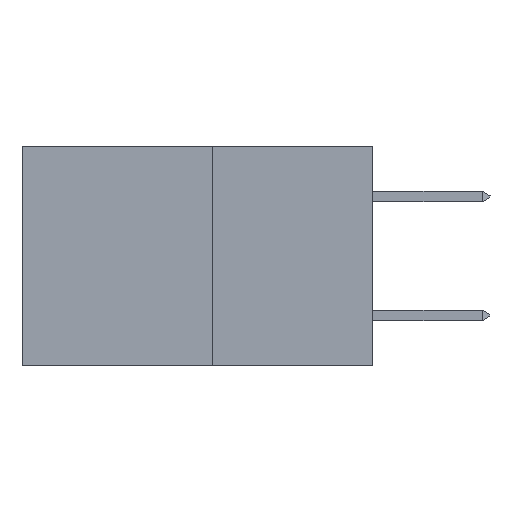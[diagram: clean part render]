
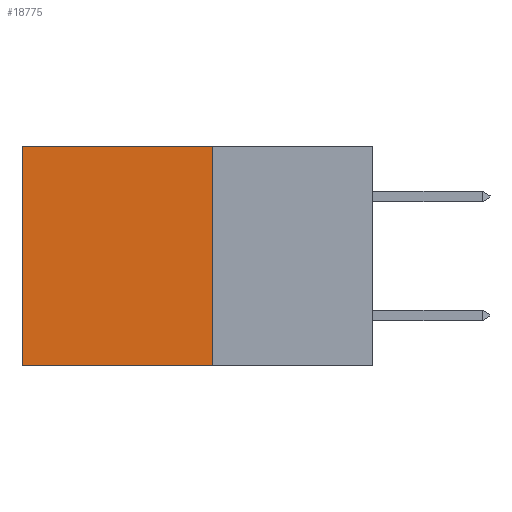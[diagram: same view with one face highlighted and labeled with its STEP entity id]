
A CAD part, left-side view. The second image highlights one B-rep face of the part: STEP entity #18775.
In plain terms, the highlighted planar face has unit normal (-1, 0, 0).
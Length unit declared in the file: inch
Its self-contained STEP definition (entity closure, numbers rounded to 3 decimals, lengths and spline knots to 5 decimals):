
#288 = AXIS2_PLACEMENT_3D ( 'NONE', #17967, #27277, #13423 ) ;
#622 = LINE ( 'NONE', #27732, #6665 ) ;
#1405 = EDGE_LOOP ( 'NONE', ( #4327, #21968, #26603, #13344 ) ) ;
#1466 = CARTESIAN_POINT ( 'NONE',  ( 0.277, 0.59, -0.37 ) ) ;
#2612 = VERTEX_POINT ( 'NONE', #11023 ) ;
#4327 = ORIENTED_EDGE ( 'NONE', *, *, #29177, .T. ) ;
#4987 = VECTOR ( 'NONE', #11175, 39.37008 ) ;
#5546 = VECTOR ( 'NONE', #26378, 39.37008 ) ;
#5677 = FACE_OUTER_BOUND ( 'NONE', #1405, .T. ) ;
#6189 = VERTEX_POINT ( 'NONE', #13771 ) ;
#6361 = VERTEX_POINT ( 'NONE', #23608 ) ;
#6665 = VECTOR ( 'NONE', #20857, 39.37008 ) ;
#9851 = DIRECTION ( 'NONE',  ( 0., 1., 0. ) ) ;
#11023 = CARTESIAN_POINT ( 'NONE',  ( 0.277, 0.27, -0.37 ) ) ;
#11074 = PLANE ( 'NONE',  #288 ) ;
#11175 = DIRECTION ( 'NONE',  ( 0., 0., -1. ) ) ;
#12424 = EDGE_CURVE ( 'NONE', #6189, #6361, #27071, .T. ) ;
#13344 = ORIENTED_EDGE ( 'NONE', *, *, #12424, .T. ) ;
#13423 = DIRECTION ( 'NONE',  ( 0., 0., -1. ) ) ;
#13771 = CARTESIAN_POINT ( 'NONE',  ( 0.277, 0.27, 0. ) ) ;
#15841 = CARTESIAN_POINT ( 'NONE',  ( 0.277, 0.27, -0.37 ) ) ;
#16478 = LINE ( 'NONE', #15841, #4987 ) ;
#17967 = CARTESIAN_POINT ( 'NONE',  ( 0.277, 0.27, -0.37 ) ) ;
#18775 = ADVANCED_FACE ( 'NONE', ( #5677 ), #11074, .F. ) ;
#18825 = EDGE_CURVE ( 'NONE', #6189, #2612, #16478, .T. ) ;
#20528 = EDGE_CURVE ( 'NONE', #2612, #22655, #24691, .T. ) ;
#20857 = DIRECTION ( 'NONE',  ( 0., 0., -1. ) ) ;
#20936 = VECTOR ( 'NONE', #9851, 39.37008 ) ;
#21968 = ORIENTED_EDGE ( 'NONE', *, *, #20528, .F. ) ;
#22655 = VERTEX_POINT ( 'NONE', #1466 ) ;
#23608 = CARTESIAN_POINT ( 'NONE',  ( 0.277, 0.59, 0. ) ) ;
#24691 = LINE ( 'NONE', #26483, #5546 ) ;
#26072 = CARTESIAN_POINT ( 'NONE',  ( 0.277, 0.27, 0. ) ) ;
#26378 = DIRECTION ( 'NONE',  ( 0., 1., 0. ) ) ;
#26483 = CARTESIAN_POINT ( 'NONE',  ( 0.277, 0.27, -0.37 ) ) ;
#26603 = ORIENTED_EDGE ( 'NONE', *, *, #18825, .F. ) ;
#27071 = LINE ( 'NONE', #26072, #20936 ) ;
#27277 = DIRECTION ( 'NONE',  ( 1., 0., 0. ) ) ;
#27732 = CARTESIAN_POINT ( 'NONE',  ( 0.277, 0.59, -0.37 ) ) ;
#29177 = EDGE_CURVE ( 'NONE', #6361, #22655, #622, .T. ) ;
